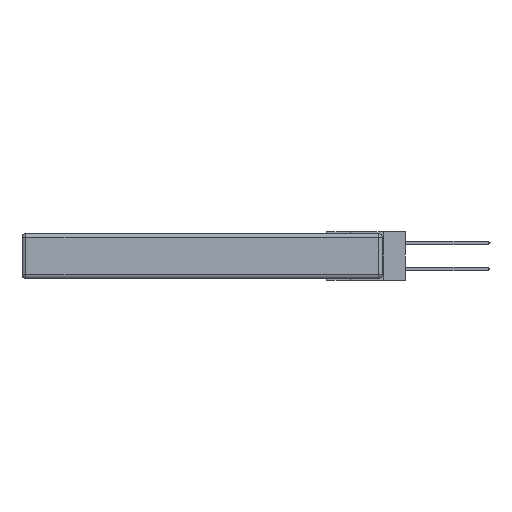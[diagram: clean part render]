
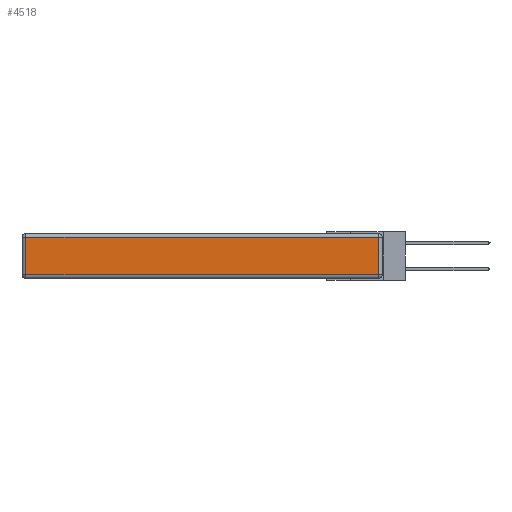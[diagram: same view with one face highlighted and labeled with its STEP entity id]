
A CAD part, left-side view. The second image highlights one B-rep face of the part: STEP entity #4518.
In plain terms, the highlighted planar face has unit normal (-1, 0, 0).
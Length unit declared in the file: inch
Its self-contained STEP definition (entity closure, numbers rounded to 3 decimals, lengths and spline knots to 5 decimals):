
#223 = DIRECTION ( 'NONE',  ( 0., 0., 1. ) ) ;
#230 = CARTESIAN_POINT ( 'NONE',  ( 0., 2.75, -0.03 ) ) ;
#531 = FACE_OUTER_BOUND ( 'NONE', #17775, .T. ) ;
#538 = CARTESIAN_POINT ( 'NONE',  ( 0., 2.72, -0.343 ) ) ;
#1040 = CARTESIAN_POINT ( 'NONE',  ( 0., 2.72, -0.313 ) ) ;
#1365 = EDGE_CURVE ( 'NONE', #17506, #16148, #18371, .T. ) ;
#2280 = DIRECTION ( 'NONE',  ( 0., 0., 1. ) ) ;
#3974 = EDGE_CURVE ( 'NONE', #6606, #17506, #19992, .T. ) ;
#4518 = ADVANCED_FACE ( 'NONE', ( #531 ), #12891, .T. ) ;
#5156 = DIRECTION ( 'NONE',  ( 0., 1., 0. ) ) ;
#5913 = LINE ( 'NONE', #538, #10669 ) ;
#6606 = VERTEX_POINT ( 'NONE', #11707 ) ;
#6843 = VECTOR ( 'NONE', #12258, 39.37008 ) ;
#7442 = CARTESIAN_POINT ( 'NONE',  ( 0., 0.03, -0.343 ) ) ;
#8049 = ORIENTED_EDGE ( 'NONE', *, *, #1365, .T. ) ;
#8095 = EDGE_CURVE ( 'NONE', #11119, #6606, #11094, .T. ) ;
#8301 = CARTESIAN_POINT ( 'NONE',  ( 0., 0., -0.343 ) ) ;
#9392 = CARTESIAN_POINT ( 'NONE',  ( 0., 0.03, -0.03 ) ) ;
#10669 = VECTOR ( 'NONE', #19411, 39.37008 ) ;
#11094 = LINE ( 'NONE', #16795, #6843 ) ;
#11119 = VERTEX_POINT ( 'NONE', #1040 ) ;
#11150 = VECTOR ( 'NONE', #5156, 39.37008 ) ;
#11707 = CARTESIAN_POINT ( 'NONE',  ( 0., 0.03, -0.313 ) ) ;
#12246 = VECTOR ( 'NONE', #2280, 39.37008 ) ;
#12258 = DIRECTION ( 'NONE',  ( 0., -1., 0. ) ) ;
#12840 = CARTESIAN_POINT ( 'NONE',  ( 0., 2.72, -0.03 ) ) ;
#12891 = PLANE ( 'NONE',  #16712 ) ;
#14515 = DIRECTION ( 'NONE',  ( -1., 0., 0. ) ) ;
#16148 = VERTEX_POINT ( 'NONE', #12840 ) ;
#16712 = AXIS2_PLACEMENT_3D ( 'NONE', #8301, #14515, #223 ) ;
#16795 = CARTESIAN_POINT ( 'NONE',  ( 0., 0., -0.313 ) ) ;
#17506 = VERTEX_POINT ( 'NONE', #9392 ) ;
#17594 = ORIENTED_EDGE ( 'NONE', *, *, #8095, .T. ) ;
#17775 = EDGE_LOOP ( 'NONE', ( #17594, #19297, #8049, #20325 ) ) ;
#17802 = EDGE_CURVE ( 'NONE', #16148, #11119, #5913, .T. ) ;
#18371 = LINE ( 'NONE', #230, #11150 ) ;
#19297 = ORIENTED_EDGE ( 'NONE', *, *, #3974, .T. ) ;
#19411 = DIRECTION ( 'NONE',  ( 0., 0., -1. ) ) ;
#19992 = LINE ( 'NONE', #7442, #12246 ) ;
#20325 = ORIENTED_EDGE ( 'NONE', *, *, #17802, .T. ) ;
